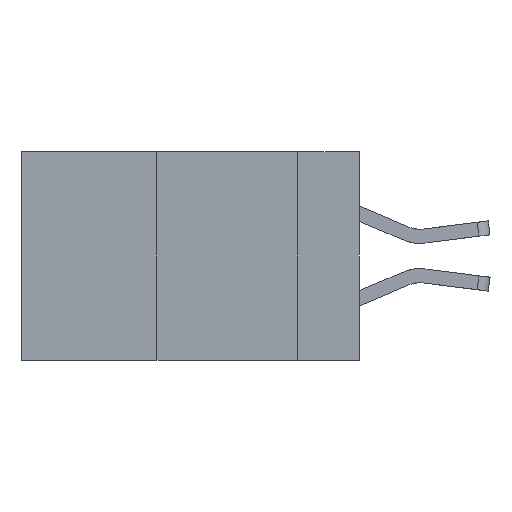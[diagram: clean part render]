
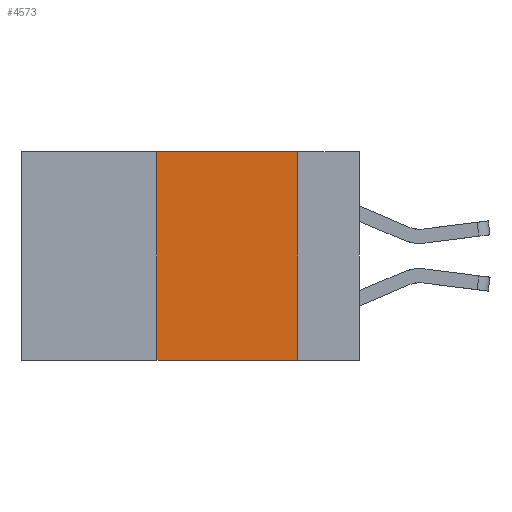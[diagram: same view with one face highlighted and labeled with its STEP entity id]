
A CAD part, left-side view. The second image highlights one B-rep face of the part: STEP entity #4573.
In plain terms, the highlighted planar face has unit normal (-1, 0, 0).
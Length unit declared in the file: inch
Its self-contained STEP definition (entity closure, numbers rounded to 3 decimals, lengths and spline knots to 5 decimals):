
#799 = VECTOR ( 'NONE', #3399, 39.37008 ) ;
#1815 = FACE_OUTER_BOUND ( 'NONE', #14817, .T. ) ;
#2314 = DIRECTION ( 'NONE',  ( 0., 0., -1. ) ) ;
#3358 = ORIENTED_EDGE ( 'NONE', *, *, #8928, .F. ) ;
#3399 = DIRECTION ( 'NONE',  ( 0., -1., 0. ) ) ;
#4344 = VERTEX_POINT ( 'NONE', #11353 ) ;
#4573 = ADVANCED_FACE ( 'NONE', ( #1815 ), #8829, .F. ) ;
#5387 = CARTESIAN_POINT ( 'NONE',  ( 0., 0.11, -0.37 ) ) ;
#5774 = LINE ( 'NONE', #9462, #799 ) ;
#6216 = AXIS2_PLACEMENT_3D ( 'NONE', #6809, #11823, #2314 ) ;
#6383 = DIRECTION ( 'NONE',  ( 0., -1., 0. ) ) ;
#6620 = DIRECTION ( 'NONE',  ( 0., 0., 1. ) ) ;
#6809 = CARTESIAN_POINT ( 'NONE',  ( 0., 0.6, 0. ) ) ;
#7044 = ORIENTED_EDGE ( 'NONE', *, *, #13647, .F. ) ;
#7150 = CARTESIAN_POINT ( 'NONE',  ( 0., 0.36, -0.37 ) ) ;
#7867 = ORIENTED_EDGE ( 'NONE', *, *, #11702, .F. ) ;
#8406 = VERTEX_POINT ( 'NONE', #13864 ) ;
#8756 = VECTOR ( 'NONE', #11343, 39.37008 ) ;
#8829 = PLANE ( 'NONE',  #6216 ) ;
#8928 = EDGE_CURVE ( 'NONE', #9580, #4344, #12675, .T. ) ;
#8939 = CARTESIAN_POINT ( 'NONE',  ( 0., 0.36, 0. ) ) ;
#9107 = LINE ( 'NONE', #13622, #8756 ) ;
#9462 = CARTESIAN_POINT ( 'NONE',  ( 0., 0.6, -0.37 ) ) ;
#9580 = VERTEX_POINT ( 'NONE', #7150 ) ;
#11073 = CARTESIAN_POINT ( 'NONE',  ( 0., 0.6, 0. ) ) ;
#11343 = DIRECTION ( 'NONE',  ( 0., 0., -1. ) ) ;
#11353 = CARTESIAN_POINT ( 'NONE',  ( 0., 0.36, 0. ) ) ;
#11702 = EDGE_CURVE ( 'NONE', #8406, #14177, #9107, .T. ) ;
#11818 = EDGE_CURVE ( 'NONE', #9580, #14177, #5774, .T. ) ;
#11823 = DIRECTION ( 'NONE',  ( 1., 0., 0. ) ) ;
#11940 = VECTOR ( 'NONE', #6620, 39.37008 ) ;
#12343 = LINE ( 'NONE', #11073, #14585 ) ;
#12675 = LINE ( 'NONE', #8939, #11940 ) ;
#13622 = CARTESIAN_POINT ( 'NONE',  ( 0., 0.11, 0. ) ) ;
#13647 = EDGE_CURVE ( 'NONE', #4344, #8406, #12343, .T. ) ;
#13864 = CARTESIAN_POINT ( 'NONE',  ( 0., 0.11, 0. ) ) ;
#14177 = VERTEX_POINT ( 'NONE', #5387 ) ;
#14585 = VECTOR ( 'NONE', #6383, 39.37008 ) ;
#14671 = ORIENTED_EDGE ( 'NONE', *, *, #11818, .T. ) ;
#14817 = EDGE_LOOP ( 'NONE', ( #7867, #7044, #3358, #14671 ) ) ;
